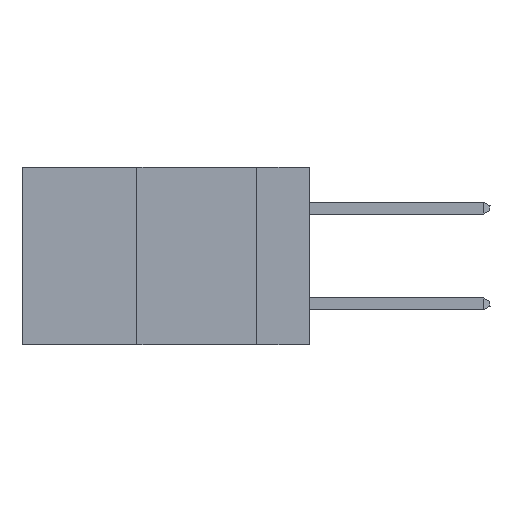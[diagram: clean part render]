
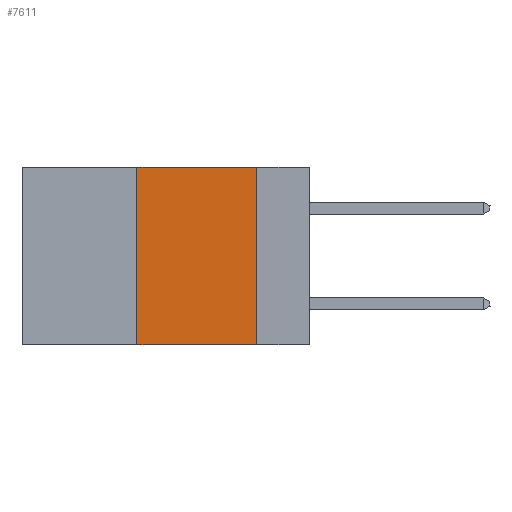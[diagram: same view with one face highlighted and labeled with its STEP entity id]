
A CAD part, left-side view. The second image highlights one B-rep face of the part: STEP entity #7611.
In plain terms, the highlighted planar face has unit normal (-1, 0, 0).
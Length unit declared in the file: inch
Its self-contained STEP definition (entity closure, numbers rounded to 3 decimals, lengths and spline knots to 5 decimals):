
#214 = DIRECTION ( 'NONE',  ( 0., -1., 0. ) ) ;
#480 = CARTESIAN_POINT ( 'NONE',  ( 0., 0.6, -0.37 ) ) ;
#525 = VECTOR ( 'NONE', #8606, 39.37008 ) ;
#748 = EDGE_CURVE ( 'NONE', #6758, #1176, #9514, .T. ) ;
#814 = CARTESIAN_POINT ( 'NONE',  ( 0., 0.36, 0. ) ) ;
#857 = EDGE_CURVE ( 'NONE', #6758, #1587, #8922, .T. ) ;
#896 = LINE ( 'NONE', #4424, #11323 ) ;
#1176 = VERTEX_POINT ( 'NONE', #6478 ) ;
#1587 = VERTEX_POINT ( 'NONE', #814 ) ;
#1893 = CARTESIAN_POINT ( 'NONE',  ( 0., 0.11, 0. ) ) ;
#2630 = VECTOR ( 'NONE', #5310, 39.37008 ) ;
#2743 = CARTESIAN_POINT ( 'NONE',  ( 0., 0.36, -0.37 ) ) ;
#2752 = EDGE_LOOP ( 'NONE', ( #10286, #3137, #10521, #6499 ) ) ;
#3041 = AXIS2_PLACEMENT_3D ( 'NONE', #5614, #7603, #3754 ) ;
#3137 = ORIENTED_EDGE ( 'NONE', *, *, #4326, .F. ) ;
#3401 = CARTESIAN_POINT ( 'NONE',  ( 0., 0.36, 0. ) ) ;
#3558 = FACE_OUTER_BOUND ( 'NONE', #2752, .T. ) ;
#3754 = DIRECTION ( 'NONE',  ( 0., 0., -1. ) ) ;
#4326 = EDGE_CURVE ( 'NONE', #1587, #9745, #6971, .T. ) ;
#4424 = CARTESIAN_POINT ( 'NONE',  ( 0., 0.11, 0. ) ) ;
#5310 = DIRECTION ( 'NONE',  ( 0., 0., 1. ) ) ;
#5614 = CARTESIAN_POINT ( 'NONE',  ( 0., 0.6, 0. ) ) ;
#5771 = PLANE ( 'NONE',  #3041 ) ;
#6087 = EDGE_CURVE ( 'NONE', #9745, #1176, #896, .T. ) ;
#6131 = VECTOR ( 'NONE', #214, 39.37008 ) ;
#6478 = CARTESIAN_POINT ( 'NONE',  ( 0., 0.11, -0.37 ) ) ;
#6499 = ORIENTED_EDGE ( 'NONE', *, *, #748, .T. ) ;
#6557 = CARTESIAN_POINT ( 'NONE',  ( 0., 0.6, 0. ) ) ;
#6758 = VERTEX_POINT ( 'NONE', #2743 ) ;
#6971 = LINE ( 'NONE', #6557, #6131 ) ;
#7603 = DIRECTION ( 'NONE',  ( 1., 0., 0. ) ) ;
#7611 = ADVANCED_FACE ( 'NONE', ( #3558 ), #5771, .F. ) ;
#8606 = DIRECTION ( 'NONE',  ( 0., -1., 0. ) ) ;
#8922 = LINE ( 'NONE', #3401, #2630 ) ;
#9514 = LINE ( 'NONE', #480, #525 ) ;
#9745 = VERTEX_POINT ( 'NONE', #1893 ) ;
#10286 = ORIENTED_EDGE ( 'NONE', *, *, #6087, .F. ) ;
#10521 = ORIENTED_EDGE ( 'NONE', *, *, #857, .F. ) ;
#10707 = DIRECTION ( 'NONE',  ( 0., 0., -1. ) ) ;
#11323 = VECTOR ( 'NONE', #10707, 39.37008 ) ;
